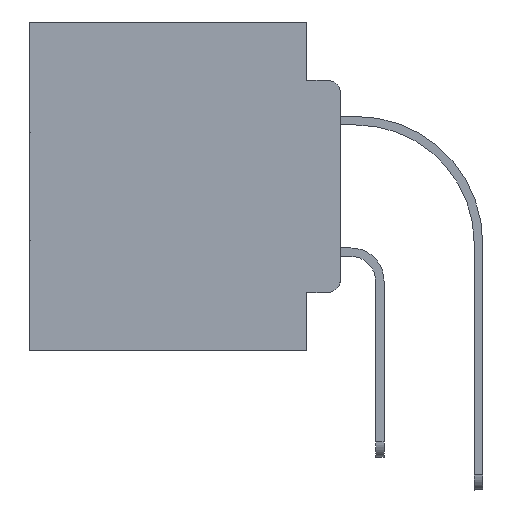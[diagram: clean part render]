
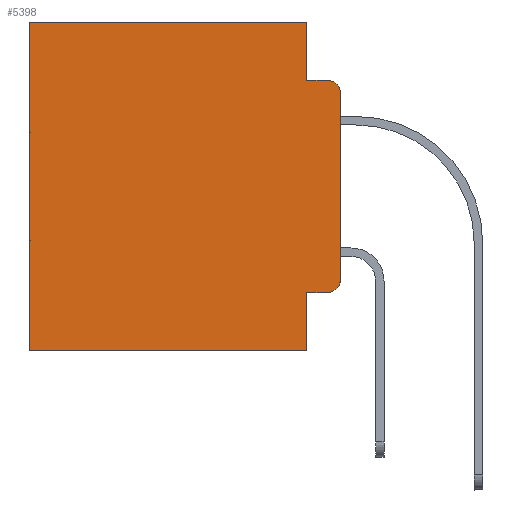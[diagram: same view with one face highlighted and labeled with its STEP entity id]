
A CAD part, left-side view. The second image highlights one B-rep face of the part: STEP entity #5398.
In plain terms, the highlighted planar face has unit normal (-1, 0, 0).
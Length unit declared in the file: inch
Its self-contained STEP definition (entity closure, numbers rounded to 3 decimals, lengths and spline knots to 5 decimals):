
#458 = DIRECTION ( 'NONE',  ( -1., 0., 0. ) ) ;
#499 = CARTESIAN_POINT ( 'NONE',  ( 0.298, 0.02, -0.1085 ) ) ;
#833 = CARTESIAN_POINT ( 'NONE',  ( 0.298, 0.051, -0.5 ) ) ;
#849 = DIRECTION ( 'NONE',  ( 0., -1., 0. ) ) ;
#1209 = EDGE_CURVE ( 'NONE', #4032, #15434, #17311, .T. ) ;
#1705 = CARTESIAN_POINT ( 'NONE',  ( 0.298, 0.051, -0.0885 ) ) ;
#2270 = CARTESIAN_POINT ( 'NONE',  ( 0.298, 0., -0.1085 ) ) ;
#2793 = CARTESIAN_POINT ( 'NONE',  ( 0.298, 0.473, 0. ) ) ;
#2856 = LINE ( 'NONE', #10603, #14351 ) ;
#3565 = DIRECTION ( 'NONE',  ( 0., 0., -1. ) ) ;
#3843 = AXIS2_PLACEMENT_3D ( 'NONE', #32966, #32466, #9778 ) ;
#3947 = EDGE_CURVE ( 'NONE', #27995, #4032, #13478, .T. ) ;
#4032 = VERTEX_POINT ( 'NONE', #4558 ) ;
#4241 = PLANE ( 'NONE',  #3843 ) ;
#4558 = CARTESIAN_POINT ( 'NONE',  ( 0.298, 0.051, -0.0885 ) ) ;
#4646 = EDGE_CURVE ( 'NONE', #29469, #24161, #13370, .T. ) ;
#4836 = CARTESIAN_POINT ( 'NONE',  ( 0.298, 0.02, -0.3915 ) ) ;
#5090 = ORIENTED_EDGE ( 'NONE', *, *, #9371, .T. ) ;
#5398 = ADVANCED_FACE ( 'NONE', ( #6924 ), #4241, .F. ) ;
#5433 = AXIS2_PLACEMENT_3D ( 'NONE', #499, #10742, #11076 ) ;
#5733 = VECTOR ( 'NONE', #6712, 39.37008 ) ;
#6398 = LINE ( 'NONE', #16816, #9330 ) ;
#6582 = EDGE_CURVE ( 'NONE', #15086, #16948, #24779, .T. ) ;
#6712 = DIRECTION ( 'NONE',  ( 0., 1., 0. ) ) ;
#6924 = FACE_OUTER_BOUND ( 'NONE', #14171, .T. ) ;
#7118 = ORIENTED_EDGE ( 'NONE', *, *, #4646, .T. ) ;
#7565 = DIRECTION ( 'NONE',  ( 0., 0., -1. ) ) ;
#8649 = CIRCLE ( 'NONE', #5433, 0.02 ) ;
#9050 = EDGE_CURVE ( 'NONE', #29786, #26278, #16324, .T. ) ;
#9330 = VECTOR ( 'NONE', #9595, 39.37008 ) ;
#9371 = EDGE_CURVE ( 'NONE', #29786, #15086, #2856, .T. ) ;
#9595 = DIRECTION ( 'NONE',  ( 0., 1., 0. ) ) ;
#9778 = DIRECTION ( 'NONE',  ( 0., 0., -1. ) ) ;
#10603 = CARTESIAN_POINT ( 'NONE',  ( 0.298, 0.051, -0.4115 ) ) ;
#10696 = DIRECTION ( 'NONE',  ( 0., 0., -1. ) ) ;
#10742 = DIRECTION ( 'NONE',  ( -1., 0., 0. ) ) ;
#11076 = DIRECTION ( 'NONE',  ( 0., 0., -1. ) ) ;
#11484 = CARTESIAN_POINT ( 'NONE',  ( 0.298, 0.02, -0.0885 ) ) ;
#11905 = CARTESIAN_POINT ( 'NONE',  ( 0.298, 0., -0.5 ) ) ;
#12675 = VERTEX_POINT ( 'NONE', #2270 ) ;
#13051 = DIRECTION ( 'NONE',  ( 0., 0., -1. ) ) ;
#13370 = LINE ( 'NONE', #2793, #21028 ) ;
#13478 = LINE ( 'NONE', #21713, #20460 ) ;
#13732 = ORIENTED_EDGE ( 'NONE', *, *, #3947, .F. ) ;
#14171 = EDGE_LOOP ( 'NONE', ( #22887, #25060, #28470, #13732, #30452, #7118, #20704, #27752, #5090, #14662 ) ) ;
#14351 = VECTOR ( 'NONE', #849, 39.37008 ) ;
#14585 = LINE ( 'NONE', #11905, #5733 ) ;
#14662 = ORIENTED_EDGE ( 'NONE', *, *, #6582, .T. ) ;
#15086 = VERTEX_POINT ( 'NONE', #26276 ) ;
#15293 = CARTESIAN_POINT ( 'NONE',  ( 0.298, 0., 0. ) ) ;
#15434 = VERTEX_POINT ( 'NONE', #11484 ) ;
#15829 = EDGE_CURVE ( 'NONE', #27995, #29469, #6398, .T. ) ;
#15831 = VECTOR ( 'NONE', #7565, 39.37008 ) ;
#16012 = CARTESIAN_POINT ( 'NONE',  ( 0.298, 0.473, 0. ) ) ;
#16324 = LINE ( 'NONE', #26587, #28309 ) ;
#16349 = CARTESIAN_POINT ( 'NONE',  ( 0.298, 0.473, -0.5 ) ) ;
#16816 = CARTESIAN_POINT ( 'NONE',  ( 0.298, 0., 0. ) ) ;
#16948 = VERTEX_POINT ( 'NONE', #21029 ) ;
#17299 = EDGE_CURVE ( 'NONE', #12675, #16948, #30602, .T. ) ;
#17311 = LINE ( 'NONE', #1705, #26586 ) ;
#20408 = EDGE_CURVE ( 'NONE', #26278, #24161, #14585, .T. ) ;
#20460 = VECTOR ( 'NONE', #29301, 39.37008 ) ;
#20704 = ORIENTED_EDGE ( 'NONE', *, *, #20408, .F. ) ;
#21028 = VECTOR ( 'NONE', #10696, 39.37008 ) ;
#21029 = CARTESIAN_POINT ( 'NONE',  ( 0.298, 0., -0.3915 ) ) ;
#21713 = CARTESIAN_POINT ( 'NONE',  ( 0.298, 0.051, 0. ) ) ;
#22755 = CARTESIAN_POINT ( 'NONE',  ( 0.298, 0.051, 0. ) ) ;
#22887 = ORIENTED_EDGE ( 'NONE', *, *, #17299, .F. ) ;
#24161 = VERTEX_POINT ( 'NONE', #16349 ) ;
#24399 = DIRECTION ( 'NONE',  ( 0., -1., 0. ) ) ;
#24779 = CIRCLE ( 'NONE', #29092, 0.02 ) ;
#25060 = ORIENTED_EDGE ( 'NONE', *, *, #26236, .T. ) ;
#26236 = EDGE_CURVE ( 'NONE', #12675, #15434, #8649, .T. ) ;
#26276 = CARTESIAN_POINT ( 'NONE',  ( 0.298, 0.02, -0.4115 ) ) ;
#26278 = VERTEX_POINT ( 'NONE', #833 ) ;
#26586 = VECTOR ( 'NONE', #24399, 39.37008 ) ;
#26587 = CARTESIAN_POINT ( 'NONE',  ( 0.298, 0.051, 0. ) ) ;
#27752 = ORIENTED_EDGE ( 'NONE', *, *, #9050, .F. ) ;
#27995 = VERTEX_POINT ( 'NONE', #22755 ) ;
#28309 = VECTOR ( 'NONE', #3565, 39.37008 ) ;
#28470 = ORIENTED_EDGE ( 'NONE', *, *, #1209, .F. ) ;
#29092 = AXIS2_PLACEMENT_3D ( 'NONE', #4836, #458, #13051 ) ;
#29301 = DIRECTION ( 'NONE',  ( 0., 0., -1. ) ) ;
#29469 = VERTEX_POINT ( 'NONE', #16012 ) ;
#29786 = VERTEX_POINT ( 'NONE', #33137 ) ;
#30452 = ORIENTED_EDGE ( 'NONE', *, *, #15829, .T. ) ;
#30602 = LINE ( 'NONE', #15293, #15831 ) ;
#32466 = DIRECTION ( 'NONE',  ( 1., 0., 0. ) ) ;
#32966 = CARTESIAN_POINT ( 'NONE',  ( 0.298, 0., 0. ) ) ;
#33137 = CARTESIAN_POINT ( 'NONE',  ( 0.298, 0.051, -0.4115 ) ) ;
